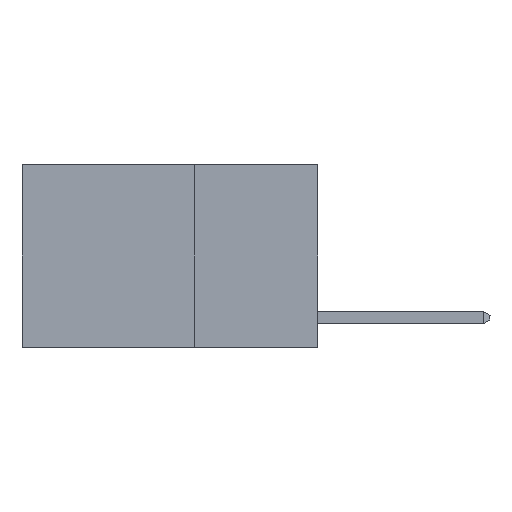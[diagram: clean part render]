
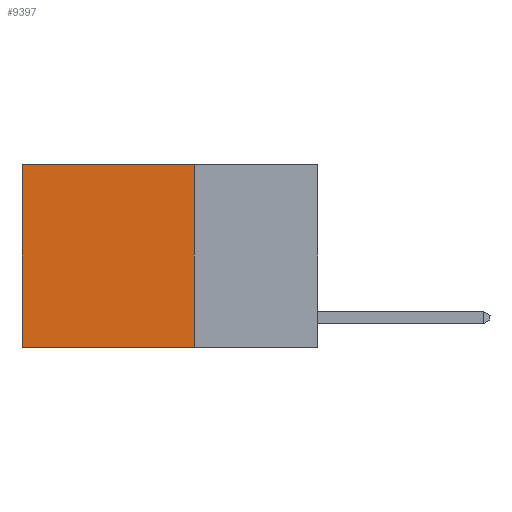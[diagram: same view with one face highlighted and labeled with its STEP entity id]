
A CAD part, left-side view. The second image highlights one B-rep face of the part: STEP entity #9397.
In plain terms, the highlighted planar face has unit normal (-1, 0, 0).
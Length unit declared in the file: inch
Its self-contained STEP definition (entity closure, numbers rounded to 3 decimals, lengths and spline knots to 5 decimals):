
#366 = CARTESIAN_POINT ( 'NONE',  ( 0.2625, 0.25, -0.37 ) ) ;
#1348 = AXIS2_PLACEMENT_3D ( 'NONE', #11290, #13869, #20513 ) ;
#1598 = VECTOR ( 'NONE', #2142, 39.37008 ) ;
#2054 = FACE_OUTER_BOUND ( 'NONE', #20806, .T. ) ;
#2142 = DIRECTION ( 'NONE',  ( 0., 0., -1. ) ) ;
#2437 = VECTOR ( 'NONE', #18338, 39.37008 ) ;
#2521 = EDGE_CURVE ( 'NONE', #20337, #4585, #16536, .T. ) ;
#2931 = DIRECTION ( 'NONE',  ( 0., 1., 0. ) ) ;
#4096 = EDGE_CURVE ( 'NONE', #4585, #13743, #29838, .T. ) ;
#4156 = ORIENTED_EDGE ( 'NONE', *, *, #2521, .T. ) ;
#4585 = VERTEX_POINT ( 'NONE', #23138 ) ;
#5016 = CARTESIAN_POINT ( 'NONE',  ( 0.2625, 0.6, 0. ) ) ;
#5962 = ORIENTED_EDGE ( 'NONE', *, *, #4096, .T. ) ;
#6694 = EDGE_CURVE ( 'NONE', #12934, #13743, #25920, .T. ) ;
#9397 = ADVANCED_FACE ( 'NONE', ( #2054 ), #16003, .F. ) ;
#11290 = CARTESIAN_POINT ( 'NONE',  ( 0.2625, 0.25, 0. ) ) ;
#12934 = VERTEX_POINT ( 'NONE', #26382 ) ;
#13743 = VERTEX_POINT ( 'NONE', #27384 ) ;
#13869 = DIRECTION ( 'NONE',  ( 1., 0., 0. ) ) ;
#14103 = DIRECTION ( 'NONE',  ( 0., 0., -1. ) ) ;
#15682 = CARTESIAN_POINT ( 'NONE',  ( 0.2625, 0.25, 0. ) ) ;
#16003 = PLANE ( 'NONE',  #1348 ) ;
#16223 = LINE ( 'NONE', #25416, #21259 ) ;
#16379 = CARTESIAN_POINT ( 'NONE',  ( 0.2625, 0.25, 0. ) ) ;
#16536 = LINE ( 'NONE', #16379, #2437 ) ;
#18338 = DIRECTION ( 'NONE',  ( 0., 1., 0. ) ) ;
#18643 = VECTOR ( 'NONE', #2931, 39.37008 ) ;
#19495 = ORIENTED_EDGE ( 'NONE', *, *, #6694, .F. ) ;
#20337 = VERTEX_POINT ( 'NONE', #15682 ) ;
#20513 = DIRECTION ( 'NONE',  ( 0., 0., -1. ) ) ;
#20806 = EDGE_LOOP ( 'NONE', ( #5962, #19495, #21976, #4156 ) ) ;
#21259 = VECTOR ( 'NONE', #14103, 39.37008 ) ;
#21976 = ORIENTED_EDGE ( 'NONE', *, *, #27570, .F. ) ;
#23138 = CARTESIAN_POINT ( 'NONE',  ( 0.2625, 0.6, 0. ) ) ;
#25416 = CARTESIAN_POINT ( 'NONE',  ( 0.2625, 0.25, 0. ) ) ;
#25920 = LINE ( 'NONE', #366, #18643 ) ;
#26382 = CARTESIAN_POINT ( 'NONE',  ( 0.2625, 0.25, -0.37 ) ) ;
#27384 = CARTESIAN_POINT ( 'NONE',  ( 0.2625, 0.6, -0.37 ) ) ;
#27570 = EDGE_CURVE ( 'NONE', #20337, #12934, #16223, .T. ) ;
#29838 = LINE ( 'NONE', #5016, #1598 ) ;
